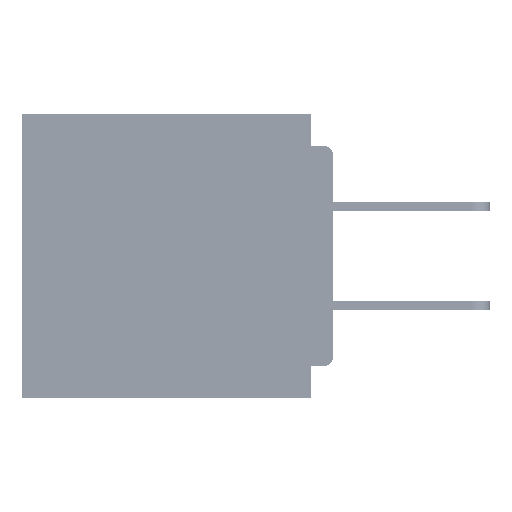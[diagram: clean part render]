
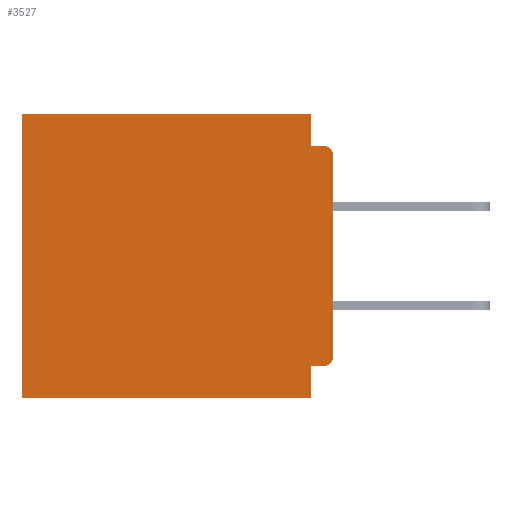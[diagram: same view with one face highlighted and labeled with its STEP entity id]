
A CAD part, left-side view. The second image highlights one B-rep face of the part: STEP entity #3527.
In plain terms, the highlighted planar face has unit normal (-1, 0, 0).
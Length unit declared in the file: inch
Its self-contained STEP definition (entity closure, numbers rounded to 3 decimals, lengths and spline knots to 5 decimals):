
#225 = VECTOR ( 'NONE', #1415, 39.37008 ) ;
#438 = DIRECTION ( 'NONE',  ( 0., 0., -1. ) ) ;
#572 = FACE_OUTER_BOUND ( 'NONE', #46308, .T. ) ;
#832 = LINE ( 'NONE', #9388, #14917 ) ;
#1415 = DIRECTION ( 'NONE',  ( 0., 0., -1. ) ) ;
#3275 = DIRECTION ( 'NONE',  ( 0., 1., 0. ) ) ;
#3527 = ADVANCED_FACE ( 'NONE', ( #572 ), #36765, .F. ) ;
#6070 = VECTOR ( 'NONE', #22708, 39.37008 ) ;
#6581 = DIRECTION ( 'NONE',  ( -1., 0., 0. ) ) ;
#7403 = CARTESIAN_POINT ( 'NONE',  ( 0.3, 0., -0.4 ) ) ;
#7407 = VECTOR ( 'NONE', #3275, 39.37008 ) ;
#8022 = ORIENTED_EDGE ( 'NONE', *, *, #26513, .T. ) ;
#8517 = VECTOR ( 'NONE', #438, 39.37008 ) ;
#9388 = CARTESIAN_POINT ( 'NONE',  ( 0.3, 0., -0.355 ) ) ;
#9892 = LINE ( 'NONE', #35239, #50611 ) ;
#10194 = LINE ( 'NONE', #64059, #8517 ) ;
#11256 = CARTESIAN_POINT ( 'NONE',  ( 0.3, 0.437, -0.4 ) ) ;
#11821 = CARTESIAN_POINT ( 'NONE',  ( 0.3, 0.031, 0. ) ) ;
#13229 = CARTESIAN_POINT ( 'NONE',  ( 0.3, 0.015, -0.355 ) ) ;
#13278 = DIRECTION ( 'NONE',  ( 0., -1., 0. ) ) ;
#14301 = LINE ( 'NONE', #11821, #225 ) ;
#14759 = ORIENTED_EDGE ( 'NONE', *, *, #41158, .T. ) ;
#14803 = CARTESIAN_POINT ( 'NONE',  ( 0.3, 0.031, 0. ) ) ;
#14917 = VECTOR ( 'NONE', #67711, 39.37008 ) ;
#16388 = CARTESIAN_POINT ( 'NONE',  ( 0.3, 0.015, -0.045 ) ) ;
#16623 = VERTEX_POINT ( 'NONE', #16388 ) ;
#17351 = CARTESIAN_POINT ( 'NONE',  ( 0.3, 0.437, -0.4 ) ) ;
#18781 = ORIENTED_EDGE ( 'NONE', *, *, #29557, .F. ) ;
#20427 = ORIENTED_EDGE ( 'NONE', *, *, #47272, .T. ) ;
#20494 = ORIENTED_EDGE ( 'NONE', *, *, #52036, .T. ) ;
#20564 = ORIENTED_EDGE ( 'NONE', *, *, #59741, .F. ) ;
#21259 = CARTESIAN_POINT ( 'NONE',  ( 0.3, 0., -0.34 ) ) ;
#21552 = LINE ( 'NONE', #24399, #7407 ) ;
#21947 = AXIS2_PLACEMENT_3D ( 'NONE', #38381, #6581, #43750 ) ;
#22615 = VERTEX_POINT ( 'NONE', #26650 ) ;
#22708 = DIRECTION ( 'NONE',  ( 0., 0., -1. ) ) ;
#24008 = VERTEX_POINT ( 'NONE', #13229 ) ;
#24399 = CARTESIAN_POINT ( 'NONE',  ( 0.3, 0., 0. ) ) ;
#24707 = CARTESIAN_POINT ( 'NONE',  ( 0.3, 0.015, -0.34 ) ) ;
#26513 = EDGE_CURVE ( 'NONE', #22615, #40973, #48475, .T. ) ;
#26650 = CARTESIAN_POINT ( 'NONE',  ( 0.3, 0.437, 0. ) ) ;
#27218 = ORIENTED_EDGE ( 'NONE', *, *, #33932, .F. ) ;
#27941 = ORIENTED_EDGE ( 'NONE', *, *, #32401, .F. ) ;
#29557 = EDGE_CURVE ( 'NONE', #43935, #40890, #9892, .T. ) ;
#30061 = DIRECTION ( 'NONE',  ( 0., 0., -1. ) ) ;
#30202 = VERTEX_POINT ( 'NONE', #57203 ) ;
#31160 = VECTOR ( 'NONE', #44585, 39.37008 ) ;
#32401 = EDGE_CURVE ( 'NONE', #49403, #52910, #14301, .T. ) ;
#32520 = DIRECTION ( 'NONE',  ( 0., 0., -1. ) ) ;
#32589 = DIRECTION ( 'NONE',  ( 1., 0., 0. ) ) ;
#33932 = EDGE_CURVE ( 'NONE', #24008, #60944, #832, .T. ) ;
#35239 = CARTESIAN_POINT ( 'NONE',  ( 0.3, 0., -0.4 ) ) ;
#35540 = LINE ( 'NONE', #61126, #63807 ) ;
#36765 = PLANE ( 'NONE',  #54930 ) ;
#36815 = CIRCLE ( 'NONE', #21947, 0.015 ) ;
#37199 = CARTESIAN_POINT ( 'NONE',  ( 0.3, 0.031, -0.355 ) ) ;
#38381 = CARTESIAN_POINT ( 'NONE',  ( 0.3, 0.015, -0.06 ) ) ;
#38961 = CARTESIAN_POINT ( 'NONE',  ( 0.3, 0., -0.4 ) ) ;
#40538 = DIRECTION ( 'NONE',  ( 0., 0., -1. ) ) ;
#40890 = VERTEX_POINT ( 'NONE', #21259 ) ;
#40973 = VERTEX_POINT ( 'NONE', #11256 ) ;
#41158 = EDGE_CURVE ( 'NONE', #24008, #40890, #67397, .T. ) ;
#43102 = EDGE_CURVE ( 'NONE', #52910, #16623, #35540, .T. ) ;
#43750 = DIRECTION ( 'NONE',  ( 0., 0., -1. ) ) ;
#43935 = VERTEX_POINT ( 'NONE', #57535 ) ;
#44585 = DIRECTION ( 'NONE',  ( 0., 1., 0. ) ) ;
#46273 = EDGE_CURVE ( 'NONE', #30202, #40973, #46957, .T. ) ;
#46308 = EDGE_LOOP ( 'NONE', ( #18781, #20427, #67844, #27941, #20494, #8022, #55405, #20564, #27218, #14759 ) ) ;
#46957 = LINE ( 'NONE', #7403, #31160 ) ;
#47272 = EDGE_CURVE ( 'NONE', #43935, #16623, #36815, .T. ) ;
#48475 = LINE ( 'NONE', #17351, #6070 ) ;
#49403 = VERTEX_POINT ( 'NONE', #14803 ) ;
#50611 = VECTOR ( 'NONE', #40538, 39.37008 ) ;
#52036 = EDGE_CURVE ( 'NONE', #49403, #22615, #21552, .T. ) ;
#52910 = VERTEX_POINT ( 'NONE', #57508 ) ;
#54930 = AXIS2_PLACEMENT_3D ( 'NONE', #38961, #32589, #32520 ) ;
#55405 = ORIENTED_EDGE ( 'NONE', *, *, #46273, .F. ) ;
#57203 = CARTESIAN_POINT ( 'NONE',  ( 0.3, 0.031, -0.4 ) ) ;
#57508 = CARTESIAN_POINT ( 'NONE',  ( 0.3, 0.031, -0.045 ) ) ;
#57535 = CARTESIAN_POINT ( 'NONE',  ( 0.3, 0., -0.06 ) ) ;
#59741 = EDGE_CURVE ( 'NONE', #60944, #30202, #10194, .T. ) ;
#60405 = AXIS2_PLACEMENT_3D ( 'NONE', #24707, #61866, #30061 ) ;
#60944 = VERTEX_POINT ( 'NONE', #37199 ) ;
#61126 = CARTESIAN_POINT ( 'NONE',  ( 0.3, 0., -0.045 ) ) ;
#61866 = DIRECTION ( 'NONE',  ( -1., 0., 0. ) ) ;
#63807 = VECTOR ( 'NONE', #13278, 39.37008 ) ;
#64059 = CARTESIAN_POINT ( 'NONE',  ( 0.3, 0.031, -0.4 ) ) ;
#67397 = CIRCLE ( 'NONE', #60405, 0.015 ) ;
#67711 = DIRECTION ( 'NONE',  ( 0., 1., 0. ) ) ;
#67844 = ORIENTED_EDGE ( 'NONE', *, *, #43102, .F. ) ;
